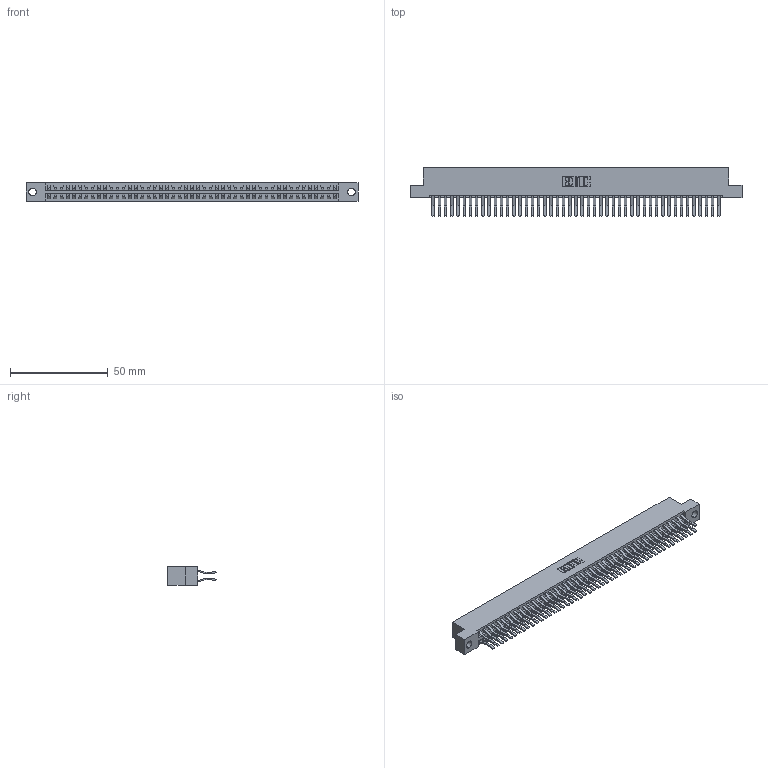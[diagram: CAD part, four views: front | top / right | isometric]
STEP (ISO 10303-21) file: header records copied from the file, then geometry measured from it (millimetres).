
FILE_DESCRIPTION (( 'STEP AP203' ), '1' );
FILE_NAME ('396-094-560-204.STEP', '2018-09-13T12:13:26', ( '' ), ( '' ), 'SwSTEP 2.0', 'SolidWorks 2016', '' );
FILE_SCHEMA (( 'CONFIG_CONTROL_DESIGN' ));
Length unit declared in the file: inch
Products named in the file (3): 396-094-560-204; 346 Part_Flush Mounting Lugs - 0.156 Dia-TH; 345-292-001_560 Tail
Assembly tree (95 placements, depth 2):
  396-094-560-204
    346 Part_Flush Mounting Lugs - 0.156 Dia-TH
    345-292-001_560 Tail  x94
Bounding box: 169.8 x 24.78 x 9.4 mm (x, y, z)
Volume: 17124.6 mm3; surface area: 25074.7 mm2
Topology: 95 solids, 95 shells, 5198 faces, 15463 edges, 10182 vertices
Faces by surface type: plane 3366, cylinder 1832
Entity records: 30091 total; most frequent: CARTESIAN_POINT 4952, ORIENTED_EDGE 4886, DIRECTION 4419, EDGE_CURVE 2443, VECTOR 2119, LINE 2119, VERTEX_POINT 1626, AXIS2_PLACEMENT_3D 1150
